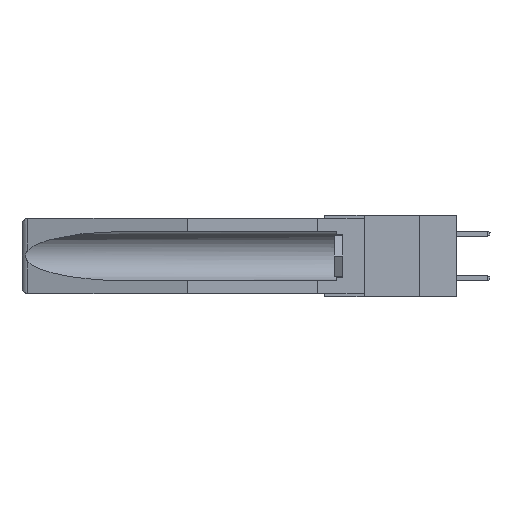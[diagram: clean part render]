
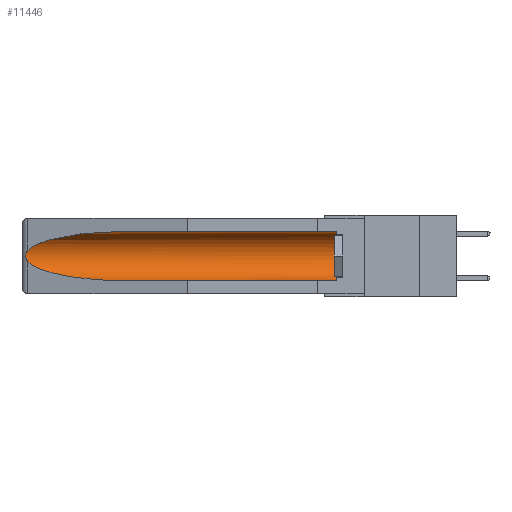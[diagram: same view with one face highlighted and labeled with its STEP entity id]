
A CAD part, left-side view. The second image highlights one B-rep face of the part: STEP entity #11446.
In plain terms, the highlighted cylindrical face has radius 2.857 mm (diameter 5.715 mm), a partial arc.
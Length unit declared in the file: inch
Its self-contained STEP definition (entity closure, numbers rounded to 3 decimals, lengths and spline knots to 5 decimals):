
#2 = CARTESIAN_POINT ( 'NONE',  ( 0.2673, 1.5327, -0.16383 ) ) ;
#325 = CARTESIAN_POINT ( 'NONE',  ( 0.26537, 1.52718, -0.14972 ) ) ;
#515 = DIRECTION ( 'NONE',  ( 0., 1., 0. ) ) ;
#551 =( BOUNDED_CURVE ( )  B_SPLINE_CURVE ( 3, ( #15629, #13720, #13874, #325 ),
 .UNSPECIFIED., .F., .F. ) 
 B_SPLINE_CURVE_WITH_KNOTS ( ( 4, 4 ),
 ( 4.71239, 6.08839 ),
 .UNSPECIFIED. ) 
 CURVE ( )  GEOMETRIC_REPRESENTATION_ITEM ( )  RATIONAL_B_SPLINE_CURVE ( ( 1., 0.848, 0.848, 1. ) ) 
 REPRESENTATION_ITEM ( '' )  );
#856 = EDGE_LOOP ( 'NONE', ( #1181, #19243, #16565, #15210, #15794, #15610 ) ) ;
#1181 = ORIENTED_EDGE ( 'NONE', *, *, #12598, .T. ) ;
#2019 = CARTESIAN_POINT ( 'NONE',  ( 0.26537, 1.52718, -0.14972 ) ) ;
#2244 = LINE ( 'NONE', #19949, #18367 ) ;
#2296 = CARTESIAN_POINT ( 'NONE',  ( 0.26537, 1.52718, -0.19328 ) ) ;
#3016 = AXIS2_PLACEMENT_3D ( 'NONE', #15937, #515, #10742 ) ;
#3451 = CARTESIAN_POINT ( 'NONE',  ( 0.26537, 1.52718, -0.19328 ) ) ;
#3526 = CARTESIAN_POINT ( 'NONE',  ( 0.26597, 1.52961, -0.15275 ) ) ;
#4021 = VERTEX_POINT ( 'NONE', #4126 ) ;
#4126 = CARTESIAN_POINT ( 'NONE',  ( 0.155, 0.126, -0.284 ) ) ;
#4645 = VERTEX_POINT ( 'NONE', #9415 ) ;
#4889 = CARTESIAN_POINT ( 'NONE',  ( 0.26597, 1.5296, -0.19026 ) ) ;
#4959 = EDGE_CURVE ( 'NONE', #4021, #21458, #16575, .T. ) ;
#6613 = CARTESIAN_POINT ( 'NONE',  ( 0.26537, 1.52718, -0.14972 ) ) ;
#6621 = FACE_OUTER_BOUND ( 'NONE', #856, .T. ) ;
#6876 = CYLINDRICAL_SURFACE ( 'NONE', #3016, 0.1125 ) ;
#7236 = CARTESIAN_POINT ( 'NONE',  ( 0.25451, 1.48313, -0.24835 ) ) ;
#7716 = CARTESIAN_POINT ( 'NONE',  ( 0.155, 0.126, -0.059 ) ) ;
#8052 = EDGE_CURVE ( 'NONE', #19097, #4645, #10898, .T. ) ;
#9109 = CARTESIAN_POINT ( 'NONE',  ( 0.155, 1.07973, -0.284 ) ) ;
#9415 = CARTESIAN_POINT ( 'NONE',  ( 0.26537, 1.52718, -0.19328 ) ) ;
#9560 = CARTESIAN_POINT ( 'NONE',  ( 0.155, 0.126, -0.1715 ) ) ;
#9700 = CIRCLE ( 'NONE', #18747, 0.1125 ) ;
#10388 = CARTESIAN_POINT ( 'NONE',  ( 0.2675, 1.53308, -0.17534 ) ) ;
#10479 = CARTESIAN_POINT ( 'NONE',  ( 0.155, 1.07973, -0.059 ) ) ;
#10742 = DIRECTION ( 'NONE',  ( 0., 0., 1. ) ) ;
#10898 = B_SPLINE_CURVE_WITH_KNOTS ( 'NONE', 3,
 ( #6613, #3526, #16976, #2, #12034, #10388, #18639, #13680, #4889, #3451 ),
 .UNSPECIFIED., .F., .F.,
 ( 4, 2, 2, 2, 4 ),
 ( 0., 0.00029, 0.00058, 0.00087, 0.00117 ),
 .UNSPECIFIED. ) ;
#11446 = ADVANCED_FACE ( 'NONE', ( #6621 ), #6876, .F. ) ;
#12034 = CARTESIAN_POINT ( 'NONE',  ( 0.2675, 1.53308, -0.16763 ) ) ;
#12187 = EDGE_CURVE ( 'NONE', #4645, #21458, #15575, .T. ) ;
#12598 = EDGE_CURVE ( 'NONE', #15512, #19097, #551, .T. ) ;
#12754 = EDGE_CURVE ( 'NONE', #22067, #15512, #2244, .T. ) ;
#13680 = CARTESIAN_POINT ( 'NONE',  ( 0.26655, 1.53094, -0.18657 ) ) ;
#13720 = CARTESIAN_POINT ( 'NONE',  ( 0.21114, 1.30732, -0.059 ) ) ;
#13874 = CARTESIAN_POINT ( 'NONE',  ( 0.25451, 1.48313, -0.09465 ) ) ;
#14327 = CARTESIAN_POINT ( 'NONE',  ( 0.155, 1.07973, -0.284 ) ) ;
#14401 = CARTESIAN_POINT ( 'NONE',  ( 0.21114, 1.30732, -0.284 ) ) ;
#14615 = DIRECTION ( 'NONE',  ( 0., 1., 0. ) ) ;
#14908 = DIRECTION ( 'NONE',  ( 0., 1., 0. ) ) ;
#15210 = ORIENTED_EDGE ( 'NONE', *, *, #4959, .F. ) ;
#15512 = VERTEX_POINT ( 'NONE', #10479 ) ;
#15575 =( BOUNDED_CURVE ( )  B_SPLINE_CURVE ( 3, ( #2296, #7236, #14401, #14327 ),
 .UNSPECIFIED., .F., .F. ) 
 B_SPLINE_CURVE_WITH_KNOTS ( ( 4, 4 ),
 ( 0.1948, 1.5708 ),
 .UNSPECIFIED. ) 
 CURVE ( )  GEOMETRIC_REPRESENTATION_ITEM ( )  RATIONAL_B_SPLINE_CURVE ( ( 1., 0.848, 0.848, 1. ) ) 
 REPRESENTATION_ITEM ( '' )  );
#15610 = ORIENTED_EDGE ( 'NONE', *, *, #12754, .T. ) ;
#15629 = CARTESIAN_POINT ( 'NONE',  ( 0.155, 1.07973, -0.059 ) ) ;
#15794 = ORIENTED_EDGE ( 'NONE', *, *, #22020, .T. ) ;
#15937 = CARTESIAN_POINT ( 'NONE',  ( 0.155, -0.30754, -0.1715 ) ) ;
#16298 = VECTOR ( 'NONE', #14908, 39.37008 ) ;
#16565 = ORIENTED_EDGE ( 'NONE', *, *, #12187, .T. ) ;
#16575 = LINE ( 'NONE', #18264, #16298 ) ;
#16976 = CARTESIAN_POINT ( 'NONE',  ( 0.26654, 1.53092, -0.15636 ) ) ;
#18264 = CARTESIAN_POINT ( 'NONE',  ( 0.155, -0.30754, -0.284 ) ) ;
#18367 = VECTOR ( 'NONE', #14615, 39.37008 ) ;
#18639 = CARTESIAN_POINT ( 'NONE',  ( 0.2673, 1.53269, -0.17917 ) ) ;
#18747 = AXIS2_PLACEMENT_3D ( 'NONE', #9560, #19613, #21599 ) ;
#19097 = VERTEX_POINT ( 'NONE', #2019 ) ;
#19243 = ORIENTED_EDGE ( 'NONE', *, *, #8052, .T. ) ;
#19613 = DIRECTION ( 'NONE',  ( 0., -1., 0. ) ) ;
#19949 = CARTESIAN_POINT ( 'NONE',  ( 0.155, -0.30754, -0.059 ) ) ;
#21458 = VERTEX_POINT ( 'NONE', #9109 ) ;
#21599 = DIRECTION ( 'NONE',  ( 0., 0., 1. ) ) ;
#22020 = EDGE_CURVE ( 'NONE', #4021, #22067, #9700, .T. ) ;
#22067 = VERTEX_POINT ( 'NONE', #7716 ) ;
